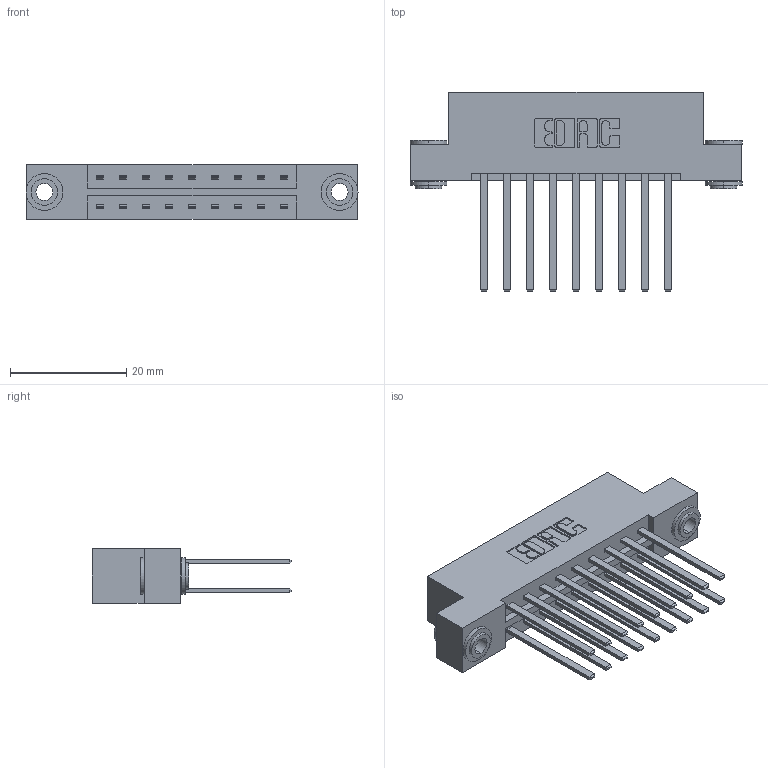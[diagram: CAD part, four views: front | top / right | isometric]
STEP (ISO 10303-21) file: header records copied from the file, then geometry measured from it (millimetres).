
FILE_DESCRIPTION (( 'STEP AP203' ), '1' );
FILE_NAME ('833-018-544-203.STEP', '2020-05-31T22:44:11', ( '' ), ( '' ), 'SwSTEP 2.0', 'SolidWorks 2020', '' );
FILE_SCHEMA (( 'CONFIG_CONTROL_DESIGN' ));
Length unit declared in the file: inch
Products named in the file (4): 345-292-001_345-293-144; 833 Part_Flush - .156 Dia - TH; 833-018-544-203; 345-250-002_345-250-002-102
Assembly tree (21 placements, depth 2):
  833-018-544-203
    833 Part_Flush - .156 Dia - TH
    345-292-001_345-293-144  x18
    345-250-002_345-250-002-102  x2
Bounding box: 57.2 x 34.3 x 9.4 mm (x, y, z)
Volume: 5803 mm3; surface area: 7539.3 mm2
Topology: 21 solids, 21 shells, 980 faces, 2853 edges, 1874 vertices
Faces by surface type: plane 656, cylinder 316, cone 8
Entity records: 10524 total; most frequent: CARTESIAN_POINT 1757, ORIENTED_EDGE 1686, DIRECTION 1589, EDGE_CURVE 843, VECTOR 695, LINE 695, VERTEX_POINT 558, AXIS2_PLACEMENT_3D 447
